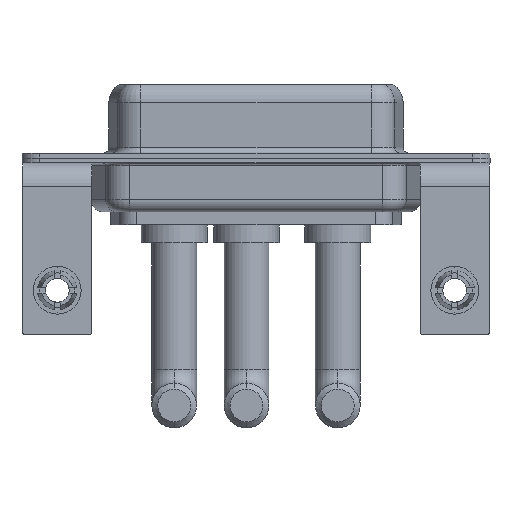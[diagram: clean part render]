
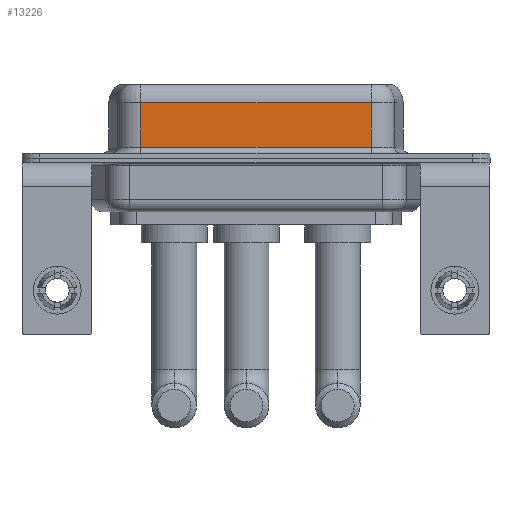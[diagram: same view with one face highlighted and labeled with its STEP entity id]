
A CAD part, front view. The second image highlights one B-rep face of the part: STEP entity #13226.
In plain terms, the highlighted planar face has unit normal (0, -1, 0).
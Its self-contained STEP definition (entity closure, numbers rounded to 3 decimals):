
#312 = FACE_OUTER_BOUND ( 'NONE', #2894, .T. ) ;
#389 = DIRECTION ( 'NONE',  ( 0., 1., 0. ) ) ;
#1402 = EDGE_CURVE ( 'NONE', #4999, #4022, #12989, .T. ) ;
#1978 = DIRECTION ( 'NONE',  ( 1., 0., 0. ) ) ;
#2039 = DIRECTION ( 'NONE',  ( -1., 0., 0. ) ) ;
#2203 = LINE ( 'NONE', #4640, #13872 ) ;
#2740 = EDGE_CURVE ( 'NONE', #13855, #4999, #15704, .T. ) ;
#2819 = ORIENTED_EDGE ( 'NONE', *, *, #13897, .F. ) ;
#2894 = EDGE_LOOP ( 'NONE', ( #2819, #14087, #11503, #5244 ) ) ;
#3556 = CARTESIAN_POINT ( 'NONE',  ( 7.013, -3.95, 0.9 ) ) ;
#4022 = VERTEX_POINT ( 'NONE', #12796 ) ;
#4080 = PLANE ( 'NONE',  #5782 ) ;
#4224 = VECTOR ( 'NONE', #8199, 1000. ) ;
#4640 = CARTESIAN_POINT ( 'NONE',  ( 26.287, -3.95, 4.65 ) ) ;
#4999 = VERTEX_POINT ( 'NONE', #3556 ) ;
#5244 = ORIENTED_EDGE ( 'NONE', *, *, #1402, .T. ) ;
#5650 = CARTESIAN_POINT ( 'NONE',  ( 7.013, -3.95, 6.4 ) ) ;
#5782 = AXIS2_PLACEMENT_3D ( 'NONE', #6679, #389, #12723 ) ;
#6679 = CARTESIAN_POINT ( 'NONE',  ( 26.287, -3.95, 6.4 ) ) ;
#7615 = VECTOR ( 'NONE', #1978, 1000. ) ;
#8122 = CARTESIAN_POINT ( 'NONE',  ( 26.287, -3.95, 6.4 ) ) ;
#8199 = DIRECTION ( 'NONE',  ( 0., 0., -1. ) ) ;
#8421 = CARTESIAN_POINT ( 'NONE',  ( 26.287, -3.95, 4.65 ) ) ;
#9150 = DIRECTION ( 'NONE',  ( 0., 0., -1. ) ) ;
#11503 = ORIENTED_EDGE ( 'NONE', *, *, #2740, .T. ) ;
#11798 = CARTESIAN_POINT ( 'NONE',  ( 7.013, -3.95, 4.65 ) ) ;
#12723 = DIRECTION ( 'NONE',  ( 0., 0., 1. ) ) ;
#12796 = CARTESIAN_POINT ( 'NONE',  ( 26.287, -3.95, 0.9 ) ) ;
#12989 = LINE ( 'NONE', #13074, #7615 ) ;
#13074 = CARTESIAN_POINT ( 'NONE',  ( 26.287, -3.95, 0.9 ) ) ;
#13226 = ADVANCED_FACE ( 'NONE', ( #312 ), #4080, .F. ) ;
#13335 = EDGE_CURVE ( 'NONE', #14489, #13855, #2203, .T. ) ;
#13855 = VERTEX_POINT ( 'NONE', #11798 ) ;
#13872 = VECTOR ( 'NONE', #2039, 1000. ) ;
#13897 = EDGE_CURVE ( 'NONE', #14489, #4022, #14438, .T. ) ;
#14087 = ORIENTED_EDGE ( 'NONE', *, *, #13335, .T. ) ;
#14438 = LINE ( 'NONE', #8122, #4224 ) ;
#14489 = VERTEX_POINT ( 'NONE', #8421 ) ;
#15213 = VECTOR ( 'NONE', #9150, 1000. ) ;
#15704 = LINE ( 'NONE', #5650, #15213 ) ;
